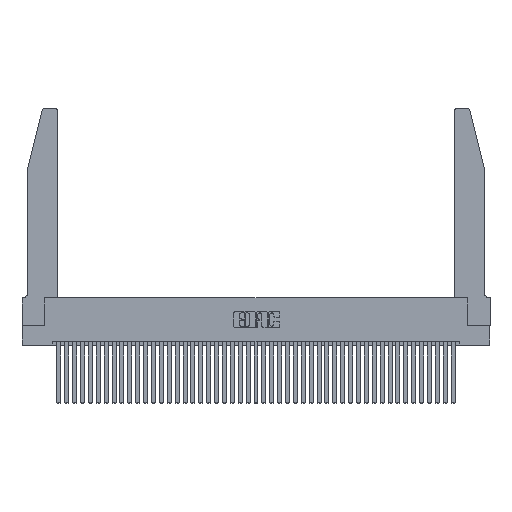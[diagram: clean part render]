
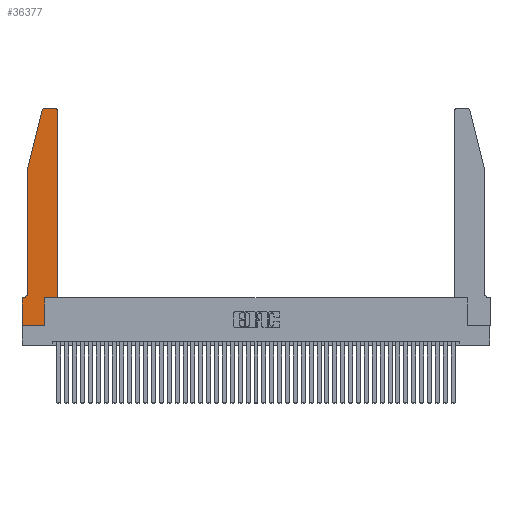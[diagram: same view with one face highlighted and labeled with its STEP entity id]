
A CAD part, top view. The second image highlights one B-rep face of the part: STEP entity #36377.
In plain terms, the highlighted planar face has unit normal (0, 0, 1).
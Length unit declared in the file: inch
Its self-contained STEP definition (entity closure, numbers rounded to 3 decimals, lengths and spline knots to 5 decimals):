
#61 = DIRECTION ( 'NONE',  ( -0.239, -0.971, 0. ) ) ;
#116 = LINE ( 'NONE', #38107, #4914 ) ;
#132 = VECTOR ( 'NONE', #39508, 39.37008 ) ;
#213 = CARTESIAN_POINT ( 'NONE',  ( 0.0755, 2., 0.37 ) ) ;
#691 = DIRECTION ( 'NONE',  ( 0., 0., 1. ) ) ;
#811 = LINE ( 'NONE', #38090, #8801 ) ;
#838 = AXIS2_PLACEMENT_3D ( 'NONE', #20976, #691, #24374 ) ;
#918 = FACE_OUTER_BOUND ( 'NONE', #1490, .T. ) ;
#1490 = EDGE_LOOP ( 'NONE', ( #2875, #41309, #18991, #15237, #20165, #1522, #9536, #29181, #8035, #37865, #31822, #19830 ) ) ;
#1522 = ORIENTED_EDGE ( 'NONE', *, *, #18370, .T. ) ;
#1794 = CARTESIAN_POINT ( 'NONE',  ( 0.284, 2.72, 0.37 ) ) ;
#2875 = ORIENTED_EDGE ( 'NONE', *, *, #39395, .T. ) ;
#3687 = VERTEX_POINT ( 'NONE', #29426 ) ;
#3750 = EDGE_CURVE ( 'NONE', #29868, #28930, #18159, .T. ) ;
#4517 = VERTEX_POINT ( 'NONE', #33547 ) ;
#4914 = VECTOR ( 'NONE', #11555, 39.37008 ) ;
#5236 = DIRECTION ( 'NONE',  ( 1., 0., 0. ) ) ;
#6199 = CARTESIAN_POINT ( 'NONE',  ( 0.2865, 0.35, 0.37 ) ) ;
#6599 = VERTEX_POINT ( 'NONE', #37300 ) ;
#6786 = CARTESIAN_POINT ( 'NONE',  ( 0., 0., 0.37 ) ) ;
#6923 = AXIS2_PLACEMENT_3D ( 'NONE', #1794, #25457, #5236 ) ;
#6968 = LINE ( 'NONE', #27129, #14858 ) ;
#7582 = CIRCLE ( 'NONE', #25350, 0.03 ) ;
#8035 = ORIENTED_EDGE ( 'NONE', *, *, #24368, .T. ) ;
#8801 = VECTOR ( 'NONE', #18324, 39.37008 ) ;
#8850 = DIRECTION ( 'NONE',  ( 0., 1., 0. ) ) ;
#9275 = CARTESIAN_POINT ( 'NONE',  ( 0.4205, 2.75, 0.37 ) ) ;
#9458 = LINE ( 'NONE', #19042, #17390 ) ;
#9536 = ORIENTED_EDGE ( 'NONE', *, *, #35562, .T. ) ;
#10308 = CARTESIAN_POINT ( 'NONE',  ( 0., 0.35, 0.37 ) ) ;
#11472 = CARTESIAN_POINT ( 'NONE',  ( 0.0055, 0.42, 0.37 ) ) ;
#11555 = DIRECTION ( 'NONE',  ( -1., 0., 0. ) ) ;
#11776 = LINE ( 'NONE', #31865, #28601 ) ;
#12222 = LINE ( 'NONE', #16425, #37789 ) ;
#13144 = EDGE_CURVE ( 'NONE', #22756, #25255, #811, .T. ) ;
#14858 = VECTOR ( 'NONE', #61, 39.37008 ) ;
#14873 = DIRECTION ( 'NONE',  ( -1., 0., 0. ) ) ;
#15047 = CARTESIAN_POINT ( 'NONE',  ( 0.4205, 2.72, 0.37 ) ) ;
#15237 = ORIENTED_EDGE ( 'NONE', *, *, #3750, .T. ) ;
#15426 = CARTESIAN_POINT ( 'NONE',  ( 0.0755, 0.42, 0.37 ) ) ;
#16377 = DIRECTION ( 'NONE',  ( -1., 0., 0. ) ) ;
#16425 = CARTESIAN_POINT ( 'NONE',  ( 0., 0., 0.37 ) ) ;
#17390 = VECTOR ( 'NONE', #8850, 39.37008 ) ;
#18159 = LINE ( 'NONE', #23027, #132 ) ;
#18324 = DIRECTION ( 'NONE',  ( 0., 1., 0. ) ) ;
#18370 = EDGE_CURVE ( 'NONE', #20064, #30520, #38301, .T. ) ;
#18418 = DIRECTION ( 'NONE',  ( 1., 0., 0. ) ) ;
#18991 = ORIENTED_EDGE ( 'NONE', *, *, #35032, .T. ) ;
#19042 = CARTESIAN_POINT ( 'NONE',  ( 0.2865, 0.35, 0.37 ) ) ;
#19479 = CIRCLE ( 'NONE', #27113, 0.07 ) ;
#19807 = DIRECTION ( 'NONE',  ( 1., 0., 0. ) ) ;
#19830 = ORIENTED_EDGE ( 'NONE', *, *, #40899, .T. ) ;
#20064 = VERTEX_POINT ( 'NONE', #38880 ) ;
#20165 = ORIENTED_EDGE ( 'NONE', *, *, #28214, .T. ) ;
#20976 = CARTESIAN_POINT ( 'NONE',  ( 0., 0.35, 0.37 ) ) ;
#21023 = CARTESIAN_POINT ( 'NONE',  ( 0.4505, 2.72, 0.37 ) ) ;
#21638 = VECTOR ( 'NONE', #26935, 39.37008 ) ;
#22038 = EDGE_CURVE ( 'NONE', #6599, #3687, #38940, .T. ) ;
#22756 = VERTEX_POINT ( 'NONE', #41366 ) ;
#22996 = CARTESIAN_POINT ( 'NONE',  ( 0.0755, 0.35, 0.37 ) ) ;
#23027 = CARTESIAN_POINT ( 'NONE',  ( 0.0755, 2., 0.37 ) ) ;
#23133 = CARTESIAN_POINT ( 'NONE',  ( 0.2865, 0., 0.37 ) ) ;
#24368 = EDGE_CURVE ( 'NONE', #33765, #33725, #9458, .T. ) ;
#24374 = DIRECTION ( 'NONE',  ( 1., 0., 0. ) ) ;
#25255 = VERTEX_POINT ( 'NONE', #21023 ) ;
#25350 = AXIS2_PLACEMENT_3D ( 'NONE', #15047, #38332, #18418 ) ;
#25457 = DIRECTION ( 'NONE',  ( 0., 0., 1. ) ) ;
#26935 = DIRECTION ( 'NONE',  ( 0., -1., 0. ) ) ;
#27113 = AXIS2_PLACEMENT_3D ( 'NONE', #11472, #34857, #14873 ) ;
#27129 = CARTESIAN_POINT ( 'NONE',  ( 0.0755, 2., 0.37 ) ) ;
#28214 = EDGE_CURVE ( 'NONE', #28930, #20064, #19479, .T. ) ;
#28601 = VECTOR ( 'NONE', #35160, 39.37008 ) ;
#28930 = VERTEX_POINT ( 'NONE', #15426 ) ;
#29181 = ORIENTED_EDGE ( 'NONE', *, *, #34913, .T. ) ;
#29426 = CARTESIAN_POINT ( 'NONE',  ( 0.25487, 2.72718, 0.37 ) ) ;
#29555 = VECTOR ( 'NONE', #16377, 39.37008 ) ;
#29868 = VERTEX_POINT ( 'NONE', #213 ) ;
#30520 = VERTEX_POINT ( 'NONE', #10308 ) ;
#31822 = ORIENTED_EDGE ( 'NONE', *, *, #13144, .T. ) ;
#31865 = CARTESIAN_POINT ( 'NONE',  ( 0.4505, 0.35, 0.37 ) ) ;
#33547 = CARTESIAN_POINT ( 'NONE',  ( 0., 0., 0.37 ) ) ;
#33725 = VERTEX_POINT ( 'NONE', #6199 ) ;
#33765 = VERTEX_POINT ( 'NONE', #23133 ) ;
#34857 = DIRECTION ( 'NONE',  ( 0., 0., -1. ) ) ;
#34913 = EDGE_CURVE ( 'NONE', #4517, #33765, #12222, .T. ) ;
#35032 = EDGE_CURVE ( 'NONE', #3687, #29868, #6968, .T. ) ;
#35160 = DIRECTION ( 'NONE',  ( 1., 0., 0. ) ) ;
#35376 = VERTEX_POINT ( 'NONE', #9275 ) ;
#35562 = EDGE_CURVE ( 'NONE', #30520, #4517, #39281, .T. ) ;
#36377 = ADVANCED_FACE ( 'NONE', ( #918 ), #37524, .T. ) ;
#37300 = CARTESIAN_POINT ( 'NONE',  ( 0.284, 2.75, 0.37 ) ) ;
#37524 = PLANE ( 'NONE',  #838 ) ;
#37789 = VECTOR ( 'NONE', #19807, 39.37008 ) ;
#37865 = ORIENTED_EDGE ( 'NONE', *, *, #40179, .T. ) ;
#38090 = CARTESIAN_POINT ( 'NONE',  ( 0.4505, 0.35, 0.37 ) ) ;
#38107 = CARTESIAN_POINT ( 'NONE',  ( 0.2605, 2.75, 0.37 ) ) ;
#38301 = LINE ( 'NONE', #22996, #29555 ) ;
#38332 = DIRECTION ( 'NONE',  ( 0., 0., 1. ) ) ;
#38880 = CARTESIAN_POINT ( 'NONE',  ( 0.0055, 0.35, 0.37 ) ) ;
#38940 = CIRCLE ( 'NONE', #6923, 0.03 ) ;
#39281 = LINE ( 'NONE', #6786, #21638 ) ;
#39395 = EDGE_CURVE ( 'NONE', #35376, #6599, #116, .T. ) ;
#39508 = DIRECTION ( 'NONE',  ( 0., -1., 0. ) ) ;
#40179 = EDGE_CURVE ( 'NONE', #33725, #22756, #11776, .T. ) ;
#40899 = EDGE_CURVE ( 'NONE', #25255, #35376, #7582, .T. ) ;
#41309 = ORIENTED_EDGE ( 'NONE', *, *, #22038, .T. ) ;
#41366 = CARTESIAN_POINT ( 'NONE',  ( 0.4505, 0.35, 0.37 ) ) ;
